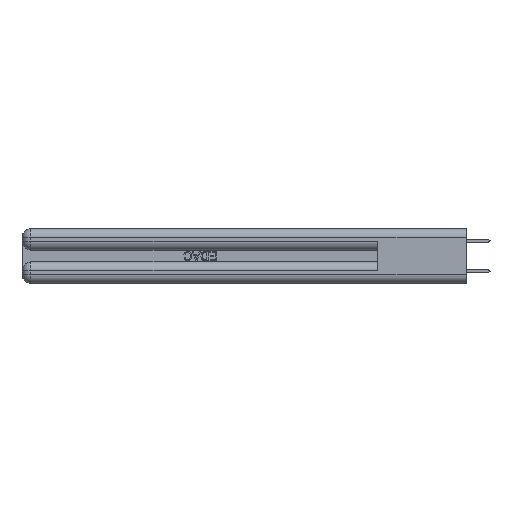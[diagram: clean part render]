
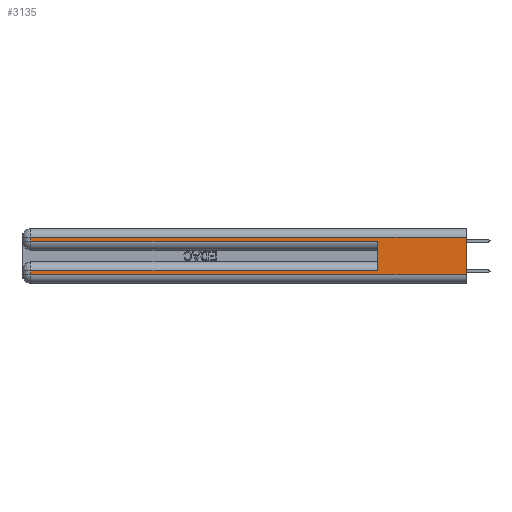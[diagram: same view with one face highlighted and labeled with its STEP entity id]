
A CAD part, left-side view. The second image highlights one B-rep face of the part: STEP entity #3135.
In plain terms, the highlighted planar face has unit normal (-1, 0, 0).
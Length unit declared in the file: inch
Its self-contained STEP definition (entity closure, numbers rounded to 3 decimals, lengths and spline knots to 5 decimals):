
#135 = EDGE_LOOP ( 'NONE', ( #29091, #33770, #17156, #17721, #2395, #38506, #37597, #26275 ) ) ;
#342 = CARTESIAN_POINT ( 'NONE',  ( 0., 0., 0.31 ) ) ;
#1298 = VECTOR ( 'NONE', #19830, 39.37008 ) ;
#1584 = CARTESIAN_POINT ( 'NONE',  ( 0., 0.6, 0.285 ) ) ;
#1940 = DIRECTION ( 'NONE',  ( 0., 0., -1. ) ) ;
#2395 = ORIENTED_EDGE ( 'NONE', *, *, #16737, .F. ) ;
#2772 = CARTESIAN_POINT ( 'NONE',  ( 0., 2.94, 0.285 ) ) ;
#3135 = ADVANCED_FACE ( 'NONE', ( #29243 ), #3515, .F. ) ;
#3515 = PLANE ( 'NONE',  #26710 ) ;
#5485 = VERTEX_POINT ( 'NONE', #1584 ) ;
#5817 = EDGE_CURVE ( 'NONE', #15844, #39844, #39859, .T. ) ;
#6234 = CARTESIAN_POINT ( 'NONE',  ( 0., 0., 0.37 ) ) ;
#7898 = CARTESIAN_POINT ( 'NONE',  ( 0., 2.94, 0.085 ) ) ;
#8074 = CARTESIAN_POINT ( 'NONE',  ( 0., 0., 0.37 ) ) ;
#8516 = LINE ( 'NONE', #13088, #32391 ) ;
#8779 = CARTESIAN_POINT ( 'NONE',  ( 0., 2.94, 0.37 ) ) ;
#9434 = LINE ( 'NONE', #8074, #22163 ) ;
#11572 = VECTOR ( 'NONE', #41221, 39.37008 ) ;
#11639 = EDGE_CURVE ( 'NONE', #13340, #15844, #38965, .T. ) ;
#11712 = EDGE_CURVE ( 'NONE', #33452, #20005, #32338, .T. ) ;
#12286 = LINE ( 'NONE', #25177, #36227 ) ;
#13088 = CARTESIAN_POINT ( 'NONE',  ( 0., 0., 0.06 ) ) ;
#13340 = VERTEX_POINT ( 'NONE', #29006 ) ;
#14687 = CARTESIAN_POINT ( 'NONE',  ( 0., 0., 0.285 ) ) ;
#15477 = VERTEX_POINT ( 'NONE', #2772 ) ;
#15844 = VERTEX_POINT ( 'NONE', #7898 ) ;
#16737 = EDGE_CURVE ( 'NONE', #13340, #5485, #12286, .T. ) ;
#17156 = ORIENTED_EDGE ( 'NONE', *, *, #29531, .T. ) ;
#17578 = VECTOR ( 'NONE', #21696, 39.37008 ) ;
#17721 = ORIENTED_EDGE ( 'NONE', *, *, #20473, .T. ) ;
#19830 = DIRECTION ( 'NONE',  ( 0., 1., 0. ) ) ;
#19896 = CARTESIAN_POINT ( 'NONE',  ( 0., 2.94, 0.06 ) ) ;
#20005 = VERTEX_POINT ( 'NONE', #29263 ) ;
#20473 = EDGE_CURVE ( 'NONE', #15477, #5485, #22697, .T. ) ;
#21260 = CARTESIAN_POINT ( 'NONE',  ( 0., 0., 0.085 ) ) ;
#21696 = DIRECTION ( 'NONE',  ( 0., 1., 0. ) ) ;
#22163 = VECTOR ( 'NONE', #1940, 39.37008 ) ;
#22697 = LINE ( 'NONE', #14687, #31830 ) ;
#23563 = DIRECTION ( 'NONE',  ( 0., 0., -1. ) ) ;
#25177 = CARTESIAN_POINT ( 'NONE',  ( 0., 0.6, 0.145 ) ) ;
#25838 = CARTESIAN_POINT ( 'NONE',  ( 0., 0., 0.06 ) ) ;
#26166 = DIRECTION ( 'NONE',  ( 0., -1., 0. ) ) ;
#26275 = ORIENTED_EDGE ( 'NONE', *, *, #41711, .T. ) ;
#26695 = CARTESIAN_POINT ( 'NONE',  ( 0., 2.94, 0.37 ) ) ;
#26710 = AXIS2_PLACEMENT_3D ( 'NONE', #6234, #39089, #33359 ) ;
#26794 = CARTESIAN_POINT ( 'NONE',  ( 0., 0., 0.31 ) ) ;
#27869 = LINE ( 'NONE', #8779, #11572 ) ;
#28155 = VECTOR ( 'NONE', #23563, 39.37008 ) ;
#29006 = CARTESIAN_POINT ( 'NONE',  ( 0., 0.6, 0.085 ) ) ;
#29091 = ORIENTED_EDGE ( 'NONE', *, *, #30788, .F. ) ;
#29243 = FACE_OUTER_BOUND ( 'NONE', #135, .T. ) ;
#29263 = CARTESIAN_POINT ( 'NONE',  ( 0., 2.94, 0.31 ) ) ;
#29531 = EDGE_CURVE ( 'NONE', #20005, #15477, #27869, .T. ) ;
#30788 = EDGE_CURVE ( 'NONE', #33452, #40335, #9434, .T. ) ;
#31830 = VECTOR ( 'NONE', #41737, 39.37008 ) ;
#32338 = LINE ( 'NONE', #342, #1298 ) ;
#32391 = VECTOR ( 'NONE', #26166, 39.37008 ) ;
#33359 = DIRECTION ( 'NONE',  ( 0., 0., -1. ) ) ;
#33452 = VERTEX_POINT ( 'NONE', #26794 ) ;
#33770 = ORIENTED_EDGE ( 'NONE', *, *, #11712, .T. ) ;
#36227 = VECTOR ( 'NONE', #38131, 39.37008 ) ;
#37597 = ORIENTED_EDGE ( 'NONE', *, *, #5817, .T. ) ;
#38131 = DIRECTION ( 'NONE',  ( 0., 0., 1. ) ) ;
#38506 = ORIENTED_EDGE ( 'NONE', *, *, #11639, .T. ) ;
#38965 = LINE ( 'NONE', #21260, #17578 ) ;
#39089 = DIRECTION ( 'NONE',  ( 1., 0., 0. ) ) ;
#39844 = VERTEX_POINT ( 'NONE', #19896 ) ;
#39859 = LINE ( 'NONE', #26695, #28155 ) ;
#40335 = VERTEX_POINT ( 'NONE', #25838 ) ;
#41221 = DIRECTION ( 'NONE',  ( 0., 0., -1. ) ) ;
#41711 = EDGE_CURVE ( 'NONE', #39844, #40335, #8516, .T. ) ;
#41737 = DIRECTION ( 'NONE',  ( 0., -1., 0. ) ) ;
